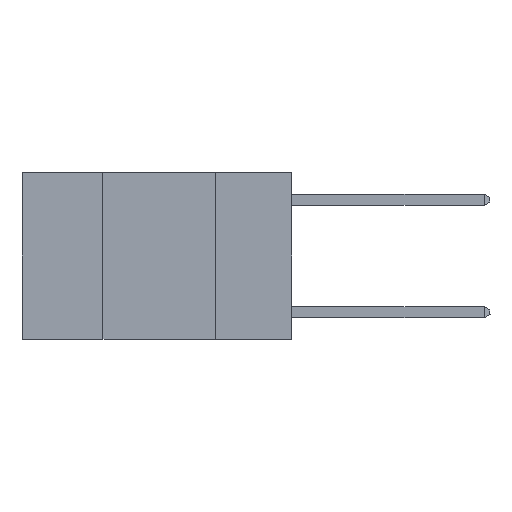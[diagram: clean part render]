
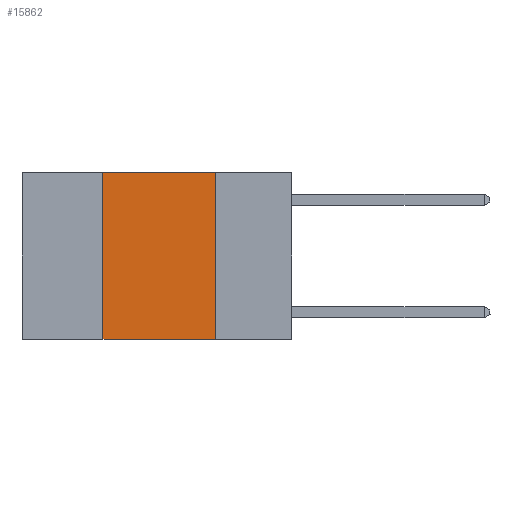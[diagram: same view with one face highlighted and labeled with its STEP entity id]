
A CAD part, left-side view. The second image highlights one B-rep face of the part: STEP entity #15862.
In plain terms, the highlighted planar face has unit normal (-1, 0, 0).
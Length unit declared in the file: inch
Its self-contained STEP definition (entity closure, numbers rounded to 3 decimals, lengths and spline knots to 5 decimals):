
#180 = VERTEX_POINT ( 'NONE', #9485 ) ;
#1682 = ORIENTED_EDGE ( 'NONE', *, *, #15746, .F. ) ;
#1708 = ORIENTED_EDGE ( 'NONE', *, *, #17253, .F. ) ;
#1991 = ORIENTED_EDGE ( 'NONE', *, *, #14558, .F. ) ;
#2213 = LINE ( 'NONE', #13270, #15999 ) ;
#2217 = CARTESIAN_POINT ( 'NONE',  ( 0., 0.17, -0.37 ) ) ;
#2228 = ORIENTED_EDGE ( 'NONE', *, *, #13365, .T. ) ;
#4055 = CARTESIAN_POINT ( 'NONE',  ( 0., 0.6, 0. ) ) ;
#4161 = LINE ( 'NONE', #6559, #14255 ) ;
#5619 = VECTOR ( 'NONE', #19809, 39.37008 ) ;
#6559 = CARTESIAN_POINT ( 'NONE',  ( 0., 0.6, 0. ) ) ;
#7248 = AXIS2_PLACEMENT_3D ( 'NONE', #4055, #20079, #9587 ) ;
#7440 = DIRECTION ( 'NONE',  ( 0., -1., 0. ) ) ;
#9277 = CARTESIAN_POINT ( 'NONE',  ( 0., 0.17, 0. ) ) ;
#9485 = CARTESIAN_POINT ( 'NONE',  ( 0., 0.42, -0.37 ) ) ;
#9587 = DIRECTION ( 'NONE',  ( 0., 0., -1. ) ) ;
#9768 = VERTEX_POINT ( 'NONE', #10197 ) ;
#10197 = CARTESIAN_POINT ( 'NONE',  ( 0., 0.17, 0. ) ) ;
#10560 = CARTESIAN_POINT ( 'NONE',  ( 0., 0.42, 0. ) ) ;
#11151 = VERTEX_POINT ( 'NONE', #10560 ) ;
#11607 = LINE ( 'NONE', #16280, #16343 ) ;
#13270 = CARTESIAN_POINT ( 'NONE',  ( 0., 0.42, 0. ) ) ;
#13365 = EDGE_CURVE ( 'NONE', #180, #17689, #11607, .T. ) ;
#14255 = VECTOR ( 'NONE', #18952, 39.37008 ) ;
#14558 = EDGE_CURVE ( 'NONE', #180, #11151, #2213, .T. ) ;
#15669 = LINE ( 'NONE', #9277, #5619 ) ;
#15746 = EDGE_CURVE ( 'NONE', #9768, #17689, #15669, .T. ) ;
#15862 = ADVANCED_FACE ( 'NONE', ( #21530 ), #18401, .F. ) ;
#15999 = VECTOR ( 'NONE', #16870, 39.37008 ) ;
#16280 = CARTESIAN_POINT ( 'NONE',  ( 0., 0.6, -0.37 ) ) ;
#16343 = VECTOR ( 'NONE', #7440, 39.37008 ) ;
#16870 = DIRECTION ( 'NONE',  ( 0., 0., 1. ) ) ;
#17253 = EDGE_CURVE ( 'NONE', #11151, #9768, #4161, .T. ) ;
#17689 = VERTEX_POINT ( 'NONE', #2217 ) ;
#18163 = EDGE_LOOP ( 'NONE', ( #1682, #1708, #1991, #2228 ) ) ;
#18401 = PLANE ( 'NONE',  #7248 ) ;
#18952 = DIRECTION ( 'NONE',  ( 0., -1., 0. ) ) ;
#19809 = DIRECTION ( 'NONE',  ( 0., 0., -1. ) ) ;
#20079 = DIRECTION ( 'NONE',  ( 1., 0., 0. ) ) ;
#21530 = FACE_OUTER_BOUND ( 'NONE', #18163, .T. ) ;
